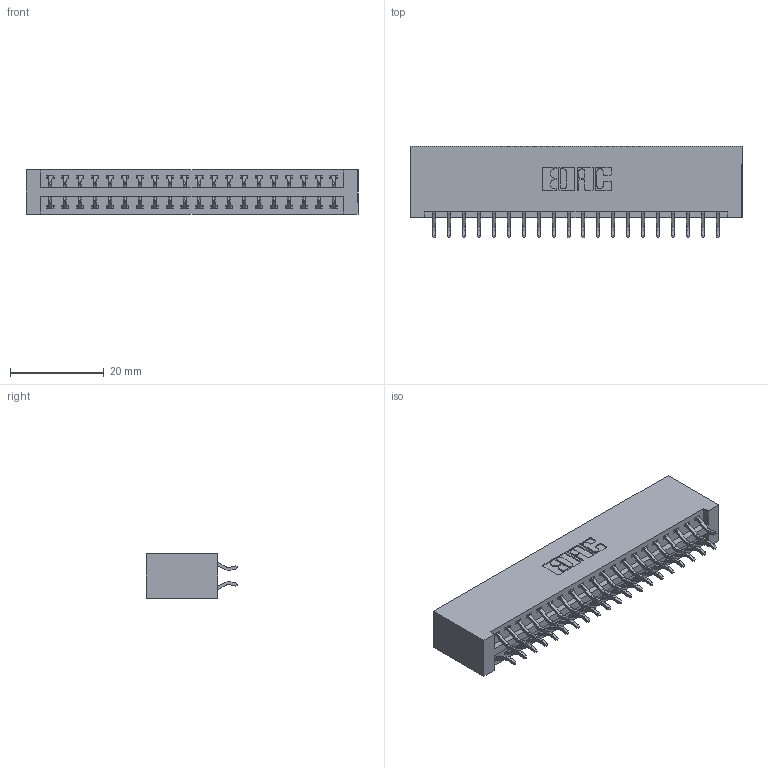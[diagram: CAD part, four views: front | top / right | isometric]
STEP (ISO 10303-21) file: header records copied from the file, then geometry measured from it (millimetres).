
FILE_DESCRIPTION (( 'STEP AP203' ), '1' );
FILE_NAME ('346-040-556-201.STEP', '2018-08-24T10:04:49', ( '' ), ( '' ), 'SwSTEP 2.0', 'SolidWorks 2016', '' );
FILE_SCHEMA (( 'CONFIG_CONTROL_DESIGN' ));
Length unit declared in the file: inch
Products named in the file (3): 345-292-001_556 Tail; 346-040-556-201; 346 Part_No Mounting Lugs
Assembly tree (41 placements, depth 2):
  346-040-556-201
    346 Part_No Mounting Lugs
    345-292-001_556 Tail  x40
Bounding box: 70.74 x 19.57 x 9.4 mm (x, y, z)
Volume: 7298.8 mm3; surface area: 9812.9 mm2
Topology: 41 solids, 41 shells, 2434 faces, 7225 edges, 4762 vertices
Faces by surface type: plane 1632, cylinder 802
Entity records: 15957 total; most frequent: CARTESIAN_POINT 2672, ORIENTED_EDGE 2594, DIRECTION 2389, EDGE_CURVE 1297, LINE 1085, VECTOR 1085, VERTEX_POINT 862, AXIS2_PLACEMENT_3D 652
